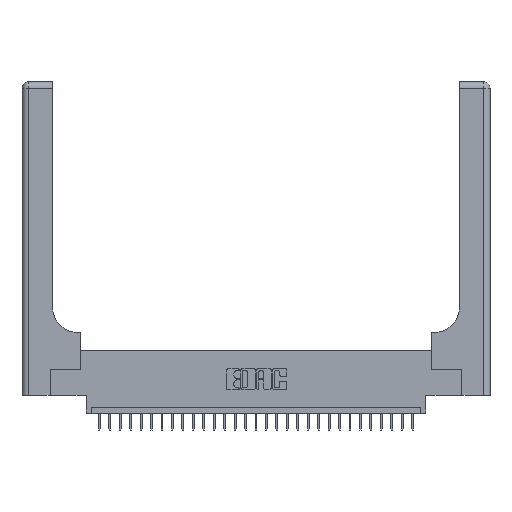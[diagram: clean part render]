
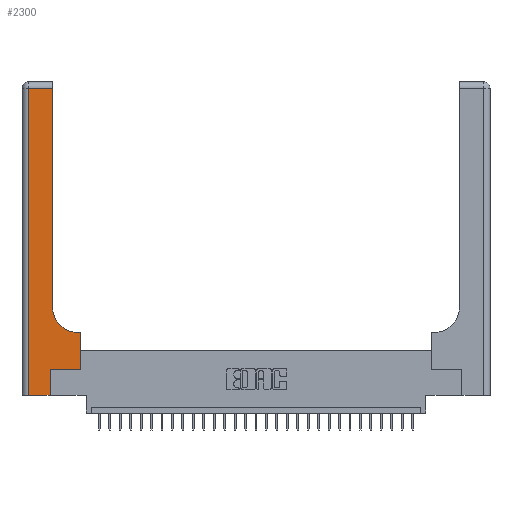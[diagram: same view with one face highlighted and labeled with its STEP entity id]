
A CAD part, top view. The second image highlights one B-rep face of the part: STEP entity #2300.
In plain terms, the highlighted planar face has unit normal (0, 0, 1).
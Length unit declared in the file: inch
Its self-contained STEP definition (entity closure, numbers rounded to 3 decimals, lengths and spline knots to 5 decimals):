
#589 = EDGE_LOOP ( 'NONE', ( #13360, #22382, #3720, #4662, #6894, #19874, #2032, #8339, #27984 ) ) ;
#970 = VECTOR ( 'NONE', #27398, 39.37008 ) ;
#987 = PLANE ( 'NONE',  #18897 ) ;
#1114 = VECTOR ( 'NONE', #13706, 39.37008 ) ;
#1126 = AXIS2_PLACEMENT_3D ( 'NONE', #3964, #10970, #8341 ) ;
#1317 = DIRECTION ( 'NONE',  ( 1., 0., 0. ) ) ;
#1454 = CARTESIAN_POINT ( 'NONE',  ( 0.269, 0., 0.37 ) ) ;
#1502 = VERTEX_POINT ( 'NONE', #19691 ) ;
#1903 = DIRECTION ( 'NONE',  ( -1., 0., 0. ) ) ;
#2032 = ORIENTED_EDGE ( 'NONE', *, *, #18330, .T. ) ;
#2079 = DIRECTION ( 'NONE',  ( 0., 1., 0. ) ) ;
#2300 = ADVANCED_FACE ( 'NONE', ( #24254 ), #987, .F. ) ;
#2314 = EDGE_CURVE ( 'NONE', #29083, #21225, #9993, .T. ) ;
#3022 = VERTEX_POINT ( 'NONE', #16033 ) ;
#3186 = VERTEX_POINT ( 'NONE', #9983 ) ;
#3720 = ORIENTED_EDGE ( 'NONE', *, *, #11941, .T. ) ;
#3964 = CARTESIAN_POINT ( 'NONE',  ( 0.5415, 0.85, 0.37 ) ) ;
#3984 = LINE ( 'NONE', #9996, #19679 ) ;
#4662 = ORIENTED_EDGE ( 'NONE', *, *, #13630, .T. ) ;
#4982 = VECTOR ( 'NONE', #26333, 39.37008 ) ;
#6501 = CARTESIAN_POINT ( 'NONE',  ( 0.269, 0., 0.37 ) ) ;
#6894 = ORIENTED_EDGE ( 'NONE', *, *, #10394, .T. ) ;
#8339 = ORIENTED_EDGE ( 'NONE', *, *, #15922, .T. ) ;
#8341 = DIRECTION ( 'NONE',  ( 1., 0., 0. ) ) ;
#8568 = CARTESIAN_POINT ( 'NONE',  ( 0.2915, 0.85, 0.37 ) ) ;
#9383 = LINE ( 'NONE', #20089, #970 ) ;
#9983 = CARTESIAN_POINT ( 'NONE',  ( 0.5585, 0.25, 0.37 ) ) ;
#9993 = CIRCLE ( 'NONE', #1126, 0.25 ) ;
#9996 = CARTESIAN_POINT ( 'NONE',  ( 0.06, 3., 0.37 ) ) ;
#10394 = EDGE_CURVE ( 'NONE', #14683, #3022, #14271, .T. ) ;
#10970 = DIRECTION ( 'NONE',  ( 0., 0., -1. ) ) ;
#11617 = CARTESIAN_POINT ( 'NONE',  ( 0.5585, 0.6, 0.37 ) ) ;
#11941 = EDGE_CURVE ( 'NONE', #28200, #25462, #3984, .T. ) ;
#12331 = LINE ( 'NONE', #20674, #19297 ) ;
#12547 = VECTOR ( 'NONE', #2079, 39.37008 ) ;
#13360 = ORIENTED_EDGE ( 'NONE', *, *, #22415, .T. ) ;
#13630 = EDGE_CURVE ( 'NONE', #25462, #14683, #9383, .T. ) ;
#13706 = DIRECTION ( 'NONE',  ( -1., 0., 0. ) ) ;
#13799 = DIRECTION ( 'NONE',  ( 0., 1., 0. ) ) ;
#14271 = LINE ( 'NONE', #6501, #27424 ) ;
#14683 = VERTEX_POINT ( 'NONE', #1454 ) ;
#14703 = VERTEX_POINT ( 'NONE', #11617 ) ;
#15167 = CARTESIAN_POINT ( 'NONE',  ( 0.5415, 0.6, 0.37 ) ) ;
#15252 = EDGE_CURVE ( 'NONE', #1502, #28200, #17140, .T. ) ;
#15256 = DIRECTION ( 'NONE',  ( -1., 0., 0. ) ) ;
#15922 = EDGE_CURVE ( 'NONE', #14703, #29083, #12331, .T. ) ;
#16033 = CARTESIAN_POINT ( 'NONE',  ( 0.269, 0.25, 0.37 ) ) ;
#17140 = LINE ( 'NONE', #29944, #1114 ) ;
#18330 = EDGE_CURVE ( 'NONE', #3186, #14703, #27876, .T. ) ;
#18897 = AXIS2_PLACEMENT_3D ( 'NONE', #25636, #19949, #15256 ) ;
#19103 = EDGE_CURVE ( 'NONE', #3022, #3186, #19457, .T. ) ;
#19297 = VECTOR ( 'NONE', #1903, 39.37008 ) ;
#19457 = LINE ( 'NONE', #21928, #26353 ) ;
#19679 = VECTOR ( 'NONE', #24184, 39.37008 ) ;
#19691 = CARTESIAN_POINT ( 'NONE',  ( 0.2915, 2.94, 0.37 ) ) ;
#19874 = ORIENTED_EDGE ( 'NONE', *, *, #19103, .T. ) ;
#19949 = DIRECTION ( 'NONE',  ( 0., 0., -1. ) ) ;
#20089 = CARTESIAN_POINT ( 'NONE',  ( 0., 0., 0.37 ) ) ;
#20674 = CARTESIAN_POINT ( 'NONE',  ( 0.2915, 0.6, 0.37 ) ) ;
#20851 = CARTESIAN_POINT ( 'NONE',  ( 0.5585, 0.25, 0.37 ) ) ;
#21072 = LINE ( 'NONE', #23694, #4982 ) ;
#21225 = VERTEX_POINT ( 'NONE', #8568 ) ;
#21928 = CARTESIAN_POINT ( 'NONE',  ( 0.269, 0.25, 0.37 ) ) ;
#22382 = ORIENTED_EDGE ( 'NONE', *, *, #15252, .T. ) ;
#22415 = EDGE_CURVE ( 'NONE', #21225, #1502, #21072, .T. ) ;
#23694 = CARTESIAN_POINT ( 'NONE',  ( 0.2915, 3., 0.37 ) ) ;
#24184 = DIRECTION ( 'NONE',  ( 0., -1., 0. ) ) ;
#24254 = FACE_OUTER_BOUND ( 'NONE', #589, .T. ) ;
#25462 = VERTEX_POINT ( 'NONE', #26658 ) ;
#25636 = CARTESIAN_POINT ( 'NONE',  ( 0., 3., 0.37 ) ) ;
#26333 = DIRECTION ( 'NONE',  ( 0., 1., 0. ) ) ;
#26353 = VECTOR ( 'NONE', #1317, 39.37008 ) ;
#26658 = CARTESIAN_POINT ( 'NONE',  ( 0.06, 0., 0.37 ) ) ;
#27398 = DIRECTION ( 'NONE',  ( 1., 0., 0. ) ) ;
#27424 = VECTOR ( 'NONE', #13799, 39.37008 ) ;
#27444 = CARTESIAN_POINT ( 'NONE',  ( 0.06, 2.94, 0.37 ) ) ;
#27876 = LINE ( 'NONE', #20851, #12547 ) ;
#27984 = ORIENTED_EDGE ( 'NONE', *, *, #2314, .T. ) ;
#28200 = VERTEX_POINT ( 'NONE', #27444 ) ;
#29083 = VERTEX_POINT ( 'NONE', #15167 ) ;
#29944 = CARTESIAN_POINT ( 'NONE',  ( 0., 2.94, 0.37 ) ) ;
